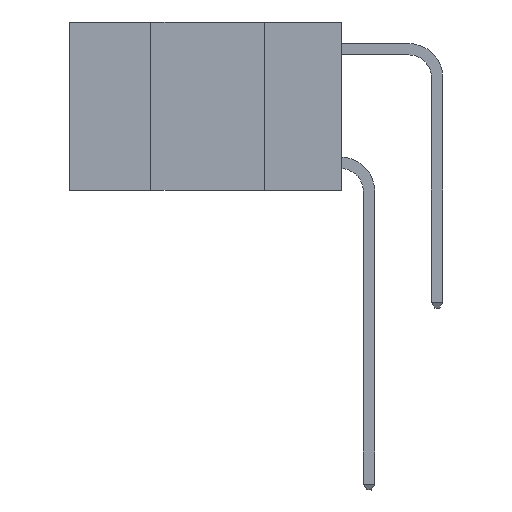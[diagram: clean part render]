
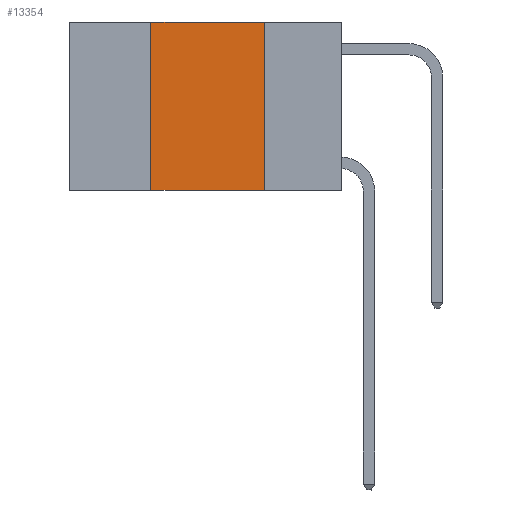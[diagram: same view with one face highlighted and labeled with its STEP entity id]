
A CAD part, left-side view. The second image highlights one B-rep face of the part: STEP entity #13354.
In plain terms, the highlighted planar face has unit normal (-1, 0, 0).
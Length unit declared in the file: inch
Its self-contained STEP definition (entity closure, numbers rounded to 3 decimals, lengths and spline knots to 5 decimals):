
#483 = EDGE_CURVE ( 'NONE', #10071, #3773, #27664, .T. ) ;
#567 = FACE_OUTER_BOUND ( 'NONE', #22960, .T. ) ;
#3773 = VERTEX_POINT ( 'NONE', #10654 ) ;
#4951 = ORIENTED_EDGE ( 'NONE', *, *, #483, .F. ) ;
#5361 = EDGE_CURVE ( 'NONE', #6949, #5616, #27742, .T. ) ;
#5616 = VERTEX_POINT ( 'NONE', #8221 ) ;
#6949 = VERTEX_POINT ( 'NONE', #8945 ) ;
#8221 = CARTESIAN_POINT ( 'NONE',  ( 0., 0.17, -0.37 ) ) ;
#8945 = CARTESIAN_POINT ( 'NONE',  ( 0., 0.42, -0.37 ) ) ;
#10071 = VERTEX_POINT ( 'NONE', #10223 ) ;
#10223 = CARTESIAN_POINT ( 'NONE',  ( 0., 0.42, 0. ) ) ;
#10291 = LINE ( 'NONE', #21149, #21218 ) ;
#10654 = CARTESIAN_POINT ( 'NONE',  ( 0., 0.17, 0. ) ) ;
#10655 = VECTOR ( 'NONE', #20261, 39.37008 ) ;
#11608 = LINE ( 'NONE', #22906, #18176 ) ;
#12801 = CARTESIAN_POINT ( 'NONE',  ( 0., 0.6, 0. ) ) ;
#13127 = DIRECTION ( 'NONE',  ( 0., 0., -1. ) ) ;
#13354 = ADVANCED_FACE ( 'NONE', ( #567 ), #22188, .F. ) ;
#13362 = ORIENTED_EDGE ( 'NONE', *, *, #5361, .T. ) ;
#15268 = EDGE_CURVE ( 'NONE', #3773, #5616, #11608, .T. ) ;
#17707 = CARTESIAN_POINT ( 'NONE',  ( 0., 0.6, 0. ) ) ;
#18176 = VECTOR ( 'NONE', #13127, 39.37008 ) ;
#19284 = CARTESIAN_POINT ( 'NONE',  ( 0., 0.6, -0.37 ) ) ;
#20261 = DIRECTION ( 'NONE',  ( 0., -1., 0. ) ) ;
#20779 = AXIS2_PLACEMENT_3D ( 'NONE', #12801, #27086, #29409 ) ;
#20896 = EDGE_CURVE ( 'NONE', #6949, #10071, #10291, .T. ) ;
#21149 = CARTESIAN_POINT ( 'NONE',  ( 0., 0.42, 0. ) ) ;
#21218 = VECTOR ( 'NONE', #25253, 39.37008 ) ;
#22188 = PLANE ( 'NONE',  #20779 ) ;
#22906 = CARTESIAN_POINT ( 'NONE',  ( 0., 0.17, 0. ) ) ;
#22960 = EDGE_LOOP ( 'NONE', ( #27092, #4951, #27305, #13362 ) ) ;
#23081 = VECTOR ( 'NONE', #26348, 39.37008 ) ;
#25253 = DIRECTION ( 'NONE',  ( 0., 0., 1. ) ) ;
#26348 = DIRECTION ( 'NONE',  ( 0., -1., 0. ) ) ;
#27086 = DIRECTION ( 'NONE',  ( 1., 0., 0. ) ) ;
#27092 = ORIENTED_EDGE ( 'NONE', *, *, #15268, .F. ) ;
#27305 = ORIENTED_EDGE ( 'NONE', *, *, #20896, .F. ) ;
#27664 = LINE ( 'NONE', #17707, #10655 ) ;
#27742 = LINE ( 'NONE', #19284, #23081 ) ;
#29409 = DIRECTION ( 'NONE',  ( 0., 0., -1. ) ) ;
